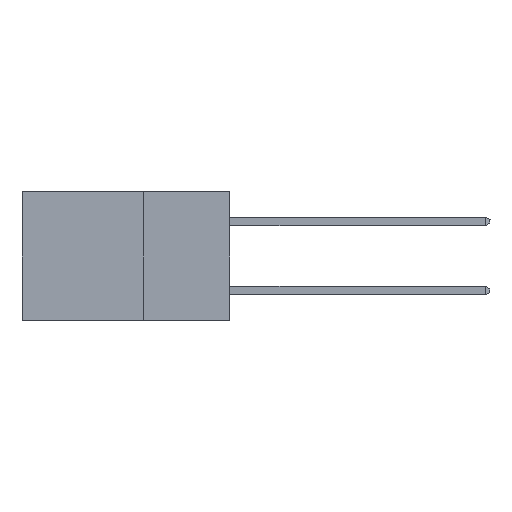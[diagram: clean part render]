
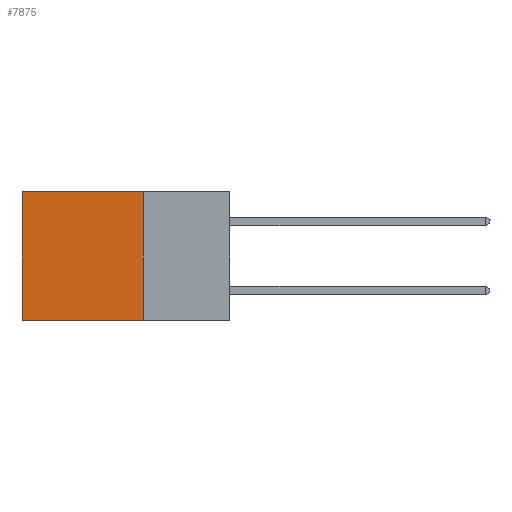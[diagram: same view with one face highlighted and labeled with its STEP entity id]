
A CAD part, left-side view. The second image highlights one B-rep face of the part: STEP entity #7875.
In plain terms, the highlighted planar face has unit normal (-1, 0, 0).
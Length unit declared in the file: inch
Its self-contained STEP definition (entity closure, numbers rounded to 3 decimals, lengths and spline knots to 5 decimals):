
#460 = LINE ( 'NONE', #9466, #5094 ) ;
#644 = EDGE_CURVE ( 'NONE', #2596, #9123, #460, .T. ) ;
#659 = FACE_OUTER_BOUND ( 'NONE', #7520, .T. ) ;
#2128 = VECTOR ( 'NONE', #3455, 39.37008 ) ;
#2392 = VERTEX_POINT ( 'NONE', #11309 ) ;
#2596 = VERTEX_POINT ( 'NONE', #9392 ) ;
#3455 = DIRECTION ( 'NONE',  ( 0., 1., 0. ) ) ;
#3526 = LINE ( 'NONE', #13893, #2128 ) ;
#3637 = LINE ( 'NONE', #10296, #13620 ) ;
#3855 = EDGE_CURVE ( 'NONE', #2596, #2392, #14193, .T. ) ;
#4983 = ORIENTED_EDGE ( 'NONE', *, *, #3855, .T. ) ;
#4994 = CARTESIAN_POINT ( 'NONE',  ( 0.2615, 0.25, 0. ) ) ;
#5094 = VECTOR ( 'NONE', #7259, 39.37008 ) ;
#5118 = CARTESIAN_POINT ( 'NONE',  ( 0.2615, 0.25, -0.37 ) ) ;
#5589 = EDGE_CURVE ( 'NONE', #9123, #14000, #3526, .T. ) ;
#5951 = DIRECTION ( 'NONE',  ( 0., 0., -1. ) ) ;
#6267 = PLANE ( 'NONE',  #9482 ) ;
#7259 = DIRECTION ( 'NONE',  ( 0., 0., -1. ) ) ;
#7520 = EDGE_LOOP ( 'NONE', ( #11835, #13991, #9655, #4983 ) ) ;
#7875 = ADVANCED_FACE ( 'NONE', ( #659 ), #6267, .F. ) ;
#9123 = VERTEX_POINT ( 'NONE', #11555 ) ;
#9392 = CARTESIAN_POINT ( 'NONE',  ( 0.2615, 0.25, 0. ) ) ;
#9466 = CARTESIAN_POINT ( 'NONE',  ( 0.2615, 0.25, -0.37 ) ) ;
#9482 = AXIS2_PLACEMENT_3D ( 'NONE', #5118, #12194, #13321 ) ;
#9655 = ORIENTED_EDGE ( 'NONE', *, *, #644, .F. ) ;
#9943 = EDGE_CURVE ( 'NONE', #2392, #14000, #3637, .T. ) ;
#10296 = CARTESIAN_POINT ( 'NONE',  ( 0.2615, 0.6, -0.37 ) ) ;
#10795 = DIRECTION ( 'NONE',  ( 0., 1., 0. ) ) ;
#11309 = CARTESIAN_POINT ( 'NONE',  ( 0.2615, 0.6, 0. ) ) ;
#11555 = CARTESIAN_POINT ( 'NONE',  ( 0.2615, 0.25, -0.37 ) ) ;
#11835 = ORIENTED_EDGE ( 'NONE', *, *, #9943, .T. ) ;
#12194 = DIRECTION ( 'NONE',  ( 1., 0., 0. ) ) ;
#13310 = VECTOR ( 'NONE', #10795, 39.37008 ) ;
#13321 = DIRECTION ( 'NONE',  ( 0., 0., -1. ) ) ;
#13620 = VECTOR ( 'NONE', #5951, 39.37008 ) ;
#13893 = CARTESIAN_POINT ( 'NONE',  ( 0.2615, 0.25, -0.37 ) ) ;
#13991 = ORIENTED_EDGE ( 'NONE', *, *, #5589, .F. ) ;
#14000 = VERTEX_POINT ( 'NONE', #14619 ) ;
#14193 = LINE ( 'NONE', #4994, #13310 ) ;
#14619 = CARTESIAN_POINT ( 'NONE',  ( 0.2615, 0.6, -0.37 ) ) ;
